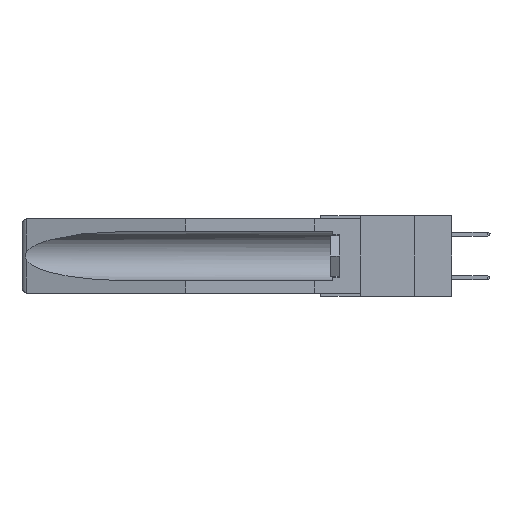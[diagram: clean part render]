
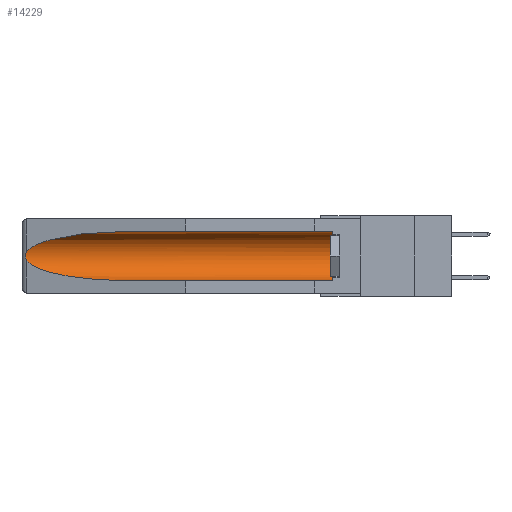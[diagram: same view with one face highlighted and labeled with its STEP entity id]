
A CAD part, left-side view. The second image highlights one B-rep face of the part: STEP entity #14229.
In plain terms, the highlighted cylindrical face has radius 2.857 mm (diameter 5.715 mm), a partial arc.
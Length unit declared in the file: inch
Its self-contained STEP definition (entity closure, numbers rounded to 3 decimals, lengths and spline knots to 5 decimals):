
#1200 = DIRECTION ( 'NONE',  ( 0., 1., 0. ) ) ;
#1303 = CARTESIAN_POINT ( 'NONE',  ( 0.26597, 1.5296, -0.19026 ) ) ;
#1427 = ORIENTED_EDGE ( 'NONE', *, *, #7108, .T. ) ;
#1456 = CARTESIAN_POINT ( 'NONE',  ( 0.25451, 1.48313, -0.09465 ) ) ;
#1463 = CARTESIAN_POINT ( 'NONE',  ( 0.155, 0.126, -0.059 ) ) ;
#1512 = AXIS2_PLACEMENT_3D ( 'NONE', #2607, #15708, #15844 ) ;
#1531 = VERTEX_POINT ( 'NONE', #4049 ) ;
#2527 = EDGE_CURVE ( 'NONE', #19169, #4505, #20979, .T. ) ;
#2607 = CARTESIAN_POINT ( 'NONE',  ( 0.155, -0.30754, -0.1715 ) ) ;
#2633 = DIRECTION ( 'NONE',  ( 0., 1., 0. ) ) ;
#2680 = CARTESIAN_POINT ( 'NONE',  ( 0.26597, 1.52961, -0.15275 ) ) ;
#2805 = VERTEX_POINT ( 'NONE', #5593 ) ;
#3007 = EDGE_CURVE ( 'NONE', #8027, #1531, #7787, .T. ) ;
#3086 = CARTESIAN_POINT ( 'NONE',  ( 0.26655, 1.53094, -0.18657 ) ) ;
#3156 = FACE_OUTER_BOUND ( 'NONE', #9070, .T. ) ;
#3418 = B_SPLINE_CURVE_WITH_KNOTS ( 'NONE', 3,
 ( #20486, #2680, #10623, #12639, #20609, #19286, #14415, #3086, #1303, #9623 ),
 .UNSPECIFIED., .F., .F.,
 ( 4, 2, 2, 2, 4 ),
 ( 0., 0.00029, 0.00058, 0.00087, 0.00117 ),
 .UNSPECIFIED. ) ;
#3523 = VERTEX_POINT ( 'NONE', #15146 ) ;
#3755 = CARTESIAN_POINT ( 'NONE',  ( 0.25451, 1.48313, -0.24835 ) ) ;
#4049 = CARTESIAN_POINT ( 'NONE',  ( 0.155, 1.07973, -0.059 ) ) ;
#4505 = VERTEX_POINT ( 'NONE', #16034 ) ;
#5037 = EDGE_CURVE ( 'NONE', #1531, #2805, #8419, .T. ) ;
#5593 = CARTESIAN_POINT ( 'NONE',  ( 0.26537, 1.52718, -0.14972 ) ) ;
#6370 = CARTESIAN_POINT ( 'NONE',  ( 0.155, 1.07973, -0.059 ) ) ;
#6984 = ORIENTED_EDGE ( 'NONE', *, *, #11722, .F. ) ;
#7108 = EDGE_CURVE ( 'NONE', #3523, #8027, #8459, .T. ) ;
#7787 = LINE ( 'NONE', #8941, #18447 ) ;
#8019 = VECTOR ( 'NONE', #1200, 39.37008 ) ;
#8027 = VERTEX_POINT ( 'NONE', #1463 ) ;
#8185 = CARTESIAN_POINT ( 'NONE',  ( 0.155, 1.07973, -0.284 ) ) ;
#8419 =( BOUNDED_CURVE ( )  B_SPLINE_CURVE ( 3, ( #6370, #16022, #1456, #12964 ),
 .UNSPECIFIED., .F., .F. ) 
 B_SPLINE_CURVE_WITH_KNOTS ( ( 4, 4 ),
 ( 4.71239, 6.08839 ),
 .UNSPECIFIED. ) 
 CURVE ( )  GEOMETRIC_REPRESENTATION_ITEM ( )  RATIONAL_B_SPLINE_CURVE ( ( 1., 0.848, 0.848, 1. ) ) 
 REPRESENTATION_ITEM ( '' )  );
#8459 = CIRCLE ( 'NONE', #15372, 0.1125 ) ;
#8941 = CARTESIAN_POINT ( 'NONE',  ( 0.155, -0.30754, -0.059 ) ) ;
#9070 = EDGE_LOOP ( 'NONE', ( #12466, #15205, #10388, #6984, #1427, #14655 ) ) ;
#9550 = CARTESIAN_POINT ( 'NONE',  ( 0.26537, 1.52718, -0.19328 ) ) ;
#9623 = CARTESIAN_POINT ( 'NONE',  ( 0.26537, 1.52718, -0.19328 ) ) ;
#10195 = DIRECTION ( 'NONE',  ( 0., 0., 1. ) ) ;
#10207 = CARTESIAN_POINT ( 'NONE',  ( 0.26537, 1.52718, -0.19328 ) ) ;
#10388 = ORIENTED_EDGE ( 'NONE', *, *, #2527, .T. ) ;
#10623 = CARTESIAN_POINT ( 'NONE',  ( 0.26654, 1.53092, -0.15636 ) ) ;
#11722 = EDGE_CURVE ( 'NONE', #3523, #4505, #12319, .T. ) ;
#12319 = LINE ( 'NONE', #19044, #8019 ) ;
#12466 = ORIENTED_EDGE ( 'NONE', *, *, #5037, .T. ) ;
#12639 = CARTESIAN_POINT ( 'NONE',  ( 0.2673, 1.5327, -0.16383 ) ) ;
#12964 = CARTESIAN_POINT ( 'NONE',  ( 0.26537, 1.52718, -0.14972 ) ) ;
#14229 = ADVANCED_FACE ( 'NONE', ( #3156 ), #17910, .F. ) ;
#14415 = CARTESIAN_POINT ( 'NONE',  ( 0.2673, 1.53269, -0.17917 ) ) ;
#14655 = ORIENTED_EDGE ( 'NONE', *, *, #3007, .T. ) ;
#14780 = DIRECTION ( 'NONE',  ( 0., -1., 0. ) ) ;
#15146 = CARTESIAN_POINT ( 'NONE',  ( 0.155, 0.126, -0.284 ) ) ;
#15205 = ORIENTED_EDGE ( 'NONE', *, *, #18144, .T. ) ;
#15372 = AXIS2_PLACEMENT_3D ( 'NONE', #19843, #14780, #10195 ) ;
#15708 = DIRECTION ( 'NONE',  ( 0., 1., 0. ) ) ;
#15844 = DIRECTION ( 'NONE',  ( 0., 0., 1. ) ) ;
#16022 = CARTESIAN_POINT ( 'NONE',  ( 0.21114, 1.30732, -0.059 ) ) ;
#16034 = CARTESIAN_POINT ( 'NONE',  ( 0.155, 1.07973, -0.284 ) ) ;
#17043 = CARTESIAN_POINT ( 'NONE',  ( 0.21114, 1.30732, -0.284 ) ) ;
#17910 = CYLINDRICAL_SURFACE ( 'NONE', #1512, 0.1125 ) ;
#18144 = EDGE_CURVE ( 'NONE', #2805, #19169, #3418, .T. ) ;
#18447 = VECTOR ( 'NONE', #2633, 39.37008 ) ;
#19044 = CARTESIAN_POINT ( 'NONE',  ( 0.155, -0.30754, -0.284 ) ) ;
#19169 = VERTEX_POINT ( 'NONE', #9550 ) ;
#19286 = CARTESIAN_POINT ( 'NONE',  ( 0.2675, 1.53308, -0.17534 ) ) ;
#19843 = CARTESIAN_POINT ( 'NONE',  ( 0.155, 0.126, -0.1715 ) ) ;
#20486 = CARTESIAN_POINT ( 'NONE',  ( 0.26537, 1.52718, -0.14972 ) ) ;
#20609 = CARTESIAN_POINT ( 'NONE',  ( 0.2675, 1.53308, -0.16763 ) ) ;
#20979 =( BOUNDED_CURVE ( )  B_SPLINE_CURVE ( 3, ( #10207, #3755, #17043, #8185 ),
 .UNSPECIFIED., .F., .F. ) 
 B_SPLINE_CURVE_WITH_KNOTS ( ( 4, 4 ),
 ( 0.1948, 1.5708 ),
 .UNSPECIFIED. ) 
 CURVE ( )  GEOMETRIC_REPRESENTATION_ITEM ( )  RATIONAL_B_SPLINE_CURVE ( ( 1., 0.848, 0.848, 1. ) ) 
 REPRESENTATION_ITEM ( '' )  );
